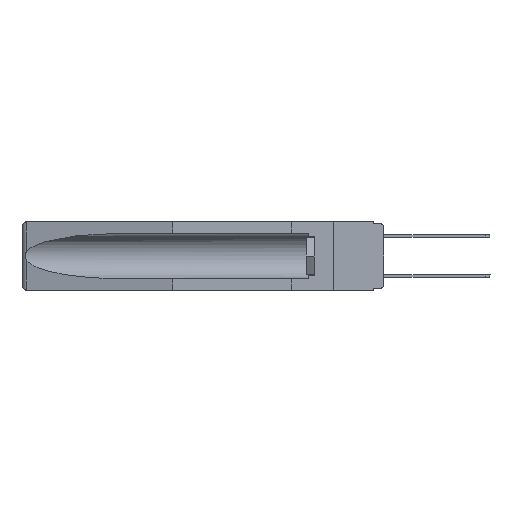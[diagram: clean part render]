
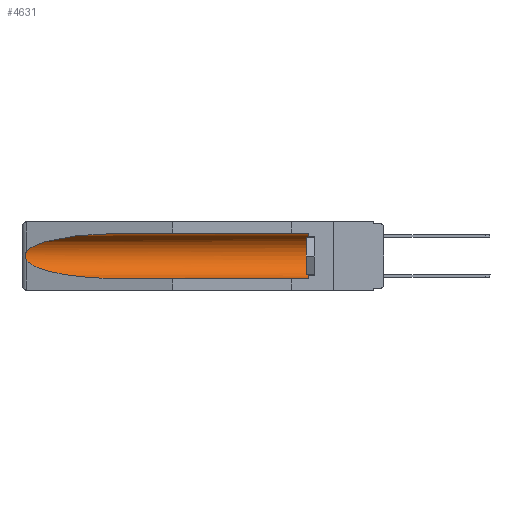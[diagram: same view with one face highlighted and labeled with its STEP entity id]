
A CAD part, left-side view. The second image highlights one B-rep face of the part: STEP entity #4631.
In plain terms, the highlighted cylindrical face has radius 2.857 mm (diameter 5.715 mm), a partial arc.
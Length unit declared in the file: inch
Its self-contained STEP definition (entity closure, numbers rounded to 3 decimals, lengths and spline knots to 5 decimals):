
#114 = CARTESIAN_POINT ( 'NONE',  ( 0.21114, 1.30732, -0.284 ) ) ;
#821 = CYLINDRICAL_SURFACE ( 'NONE', #19833, 0.1125 ) ;
#1431 = CARTESIAN_POINT ( 'NONE',  ( 0.26537, 1.52718, -0.19328 ) ) ;
#1753 = CARTESIAN_POINT ( 'NONE',  ( 0.155, 0.126, -0.1715 ) ) ;
#1947 = ORIENTED_EDGE ( 'NONE', *, *, #16035, .F. ) ;
#2175 = CARTESIAN_POINT ( 'NONE',  ( 0.2675, 1.53308, -0.17534 ) ) ;
#2291 = CARTESIAN_POINT ( 'NONE',  ( 0.26537, 1.52718, -0.19328 ) ) ;
#2628 = EDGE_CURVE ( 'NONE', #5118, #11009, #6326, .T. ) ;
#2938 = LINE ( 'NONE', #15205, #8004 ) ;
#3575 = DIRECTION ( 'NONE',  ( 0., 0., 1. ) ) ;
#3650 = FACE_OUTER_BOUND ( 'NONE', #6519, .T. ) ;
#3794 = CARTESIAN_POINT ( 'NONE',  ( 0.26655, 1.53094, -0.18657 ) ) ;
#4631 = ADVANCED_FACE ( 'NONE', ( #3650 ), #821, .F. ) ;
#4667 = CARTESIAN_POINT ( 'NONE',  ( 0.25451, 1.48313, -0.24835 ) ) ;
#4707 = AXIS2_PLACEMENT_3D ( 'NONE', #1753, #14235, #3575 ) ;
#4784 = ORIENTED_EDGE ( 'NONE', *, *, #2628, .T. ) ;
#5118 = VERTEX_POINT ( 'NONE', #11212 ) ;
#5458 = CARTESIAN_POINT ( 'NONE',  ( 0.26597, 1.52961, -0.15275 ) ) ;
#5485 = CARTESIAN_POINT ( 'NONE',  ( 0.26537, 1.52718, -0.14972 ) ) ;
#6233 = ORIENTED_EDGE ( 'NONE', *, *, #12556, .T. ) ;
#6326 = CIRCLE ( 'NONE', #4707, 0.1125 ) ;
#6519 = EDGE_LOOP ( 'NONE', ( #6233, #17212, #7870, #1947, #4784, #15893 ) ) ;
#6829 = CARTESIAN_POINT ( 'NONE',  ( 0.2673, 1.53269, -0.17917 ) ) ;
#6955 = VERTEX_POINT ( 'NONE', #14468 ) ;
#6982 = CARTESIAN_POINT ( 'NONE',  ( 0.155, -0.30754, -0.1715 ) ) ;
#7870 = ORIENTED_EDGE ( 'NONE', *, *, #16020, .T. ) ;
#8004 = VECTOR ( 'NONE', #10725, 39.37008 ) ;
#8029 = VECTOR ( 'NONE', #18845, 39.37008 ) ;
#8207 = LINE ( 'NONE', #14228, #8029 ) ;
#8789 = CARTESIAN_POINT ( 'NONE',  ( 0.155, 1.07973, -0.059 ) ) ;
#8805 = VERTEX_POINT ( 'NONE', #15681 ) ;
#9017 = CARTESIAN_POINT ( 'NONE',  ( 0.155, 0.126, -0.059 ) ) ;
#9807 = DIRECTION ( 'NONE',  ( 0., 1., 0. ) ) ;
#10072 = CARTESIAN_POINT ( 'NONE',  ( 0.2675, 1.53308, -0.16763 ) ) ;
#10206 = CARTESIAN_POINT ( 'NONE',  ( 0.21114, 1.30732, -0.059 ) ) ;
#10725 = DIRECTION ( 'NONE',  ( 0., 1., 0. ) ) ;
#10850 =( BOUNDED_CURVE ( )  B_SPLINE_CURVE ( 3, ( #8789, #10206, #13301, #5485 ),
 .UNSPECIFIED., .F., .T. ) 
 B_SPLINE_CURVE_WITH_KNOTS ( ( 4, 4 ),
 ( 4.71239, 6.08839 ),
 .UNSPECIFIED. ) 
 CURVE ( )  GEOMETRIC_REPRESENTATION_ITEM ( )  RATIONAL_B_SPLINE_CURVE ( ( 1., 0.848, 0.848, 1. ) ) 
 REPRESENTATION_ITEM ( '' )  );
#11009 = VERTEX_POINT ( 'NONE', #9017 ) ;
#11212 = CARTESIAN_POINT ( 'NONE',  ( 0.155, 0.126, -0.284 ) ) ;
#11261 = CARTESIAN_POINT ( 'NONE',  ( 0.26537, 1.52718, -0.19328 ) ) ;
#11581 = CARTESIAN_POINT ( 'NONE',  ( 0.26654, 1.53092, -0.15636 ) ) ;
#12556 = EDGE_CURVE ( 'NONE', #6955, #8805, #10850, .T. ) ;
#12869 =( BOUNDED_CURVE ( )  B_SPLINE_CURVE ( 3, ( #1431, #4667, #114, #19830 ),
 .UNSPECIFIED., .F., .F. ) 
 B_SPLINE_CURVE_WITH_KNOTS ( ( 4, 4 ),
 ( 0.1948, 1.5708 ),
 .UNSPECIFIED. ) 
 CURVE ( )  GEOMETRIC_REPRESENTATION_ITEM ( )  RATIONAL_B_SPLINE_CURVE ( ( 1., 0.848, 0.848, 1. ) ) 
 REPRESENTATION_ITEM ( '' )  );
#13085 = EDGE_CURVE ( 'NONE', #8805, #15388, #19776, .T. ) ;
#13301 = CARTESIAN_POINT ( 'NONE',  ( 0.25451, 1.48313, -0.09465 ) ) ;
#14228 = CARTESIAN_POINT ( 'NONE',  ( 0.155, -0.30754, -0.059 ) ) ;
#14235 = DIRECTION ( 'NONE',  ( 0., -1., 0. ) ) ;
#14359 = CARTESIAN_POINT ( 'NONE',  ( 0.155, 1.07973, -0.284 ) ) ;
#14468 = CARTESIAN_POINT ( 'NONE',  ( 0.155, 1.07973, -0.059 ) ) ;
#15205 = CARTESIAN_POINT ( 'NONE',  ( 0.155, -0.30754, -0.284 ) ) ;
#15388 = VERTEX_POINT ( 'NONE', #2291 ) ;
#15681 = CARTESIAN_POINT ( 'NONE',  ( 0.26537, 1.52718, -0.14972 ) ) ;
#15893 = ORIENTED_EDGE ( 'NONE', *, *, #18383, .T. ) ;
#16003 = DIRECTION ( 'NONE',  ( 0., 0., 1. ) ) ;
#16020 = EDGE_CURVE ( 'NONE', #15388, #17162, #12869, .T. ) ;
#16035 = EDGE_CURVE ( 'NONE', #5118, #17162, #2938, .T. ) ;
#17162 = VERTEX_POINT ( 'NONE', #14359 ) ;
#17212 = ORIENTED_EDGE ( 'NONE', *, *, #13085, .T. ) ;
#17263 = CARTESIAN_POINT ( 'NONE',  ( 0.26597, 1.5296, -0.19026 ) ) ;
#17681 = CARTESIAN_POINT ( 'NONE',  ( 0.2673, 1.5327, -0.16383 ) ) ;
#18383 = EDGE_CURVE ( 'NONE', #11009, #6955, #8207, .T. ) ;
#18845 = DIRECTION ( 'NONE',  ( 0., 1., 0. ) ) ;
#19197 = CARTESIAN_POINT ( 'NONE',  ( 0.26537, 1.52718, -0.14972 ) ) ;
#19776 = B_SPLINE_CURVE_WITH_KNOTS ( 'NONE', 3,
 ( #19197, #5458, #11581, #17681, #10072, #2175, #6829, #3794, #17263, #11261 ),
 .UNSPECIFIED., .F., .F.,
 ( 4, 2, 2, 2, 4 ),
 ( 0., 0.00029, 0.00058, 0.00087, 0.00117 ),
 .UNSPECIFIED. ) ;
#19830 = CARTESIAN_POINT ( 'NONE',  ( 0.155, 1.07973, -0.284 ) ) ;
#19833 = AXIS2_PLACEMENT_3D ( 'NONE', #6982, #9807, #16003 ) ;
